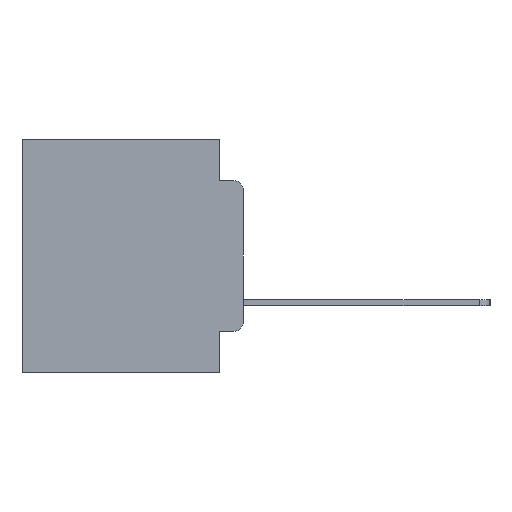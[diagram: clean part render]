
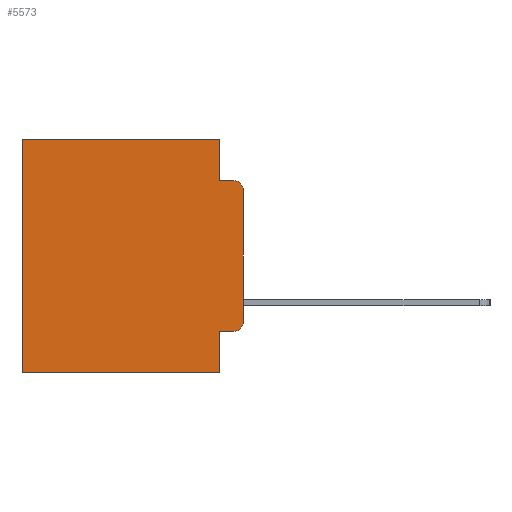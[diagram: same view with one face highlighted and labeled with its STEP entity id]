
A CAD part, left-side view. The second image highlights one B-rep face of the part: STEP entity #5573.
In plain terms, the highlighted planar face has unit normal (-1, 0, 0).
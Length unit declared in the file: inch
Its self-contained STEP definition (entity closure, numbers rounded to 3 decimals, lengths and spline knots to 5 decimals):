
#157 = CARTESIAN_POINT ( 'NONE',  ( 0.298, 0.051, 0. ) ) ;
#373 = DIRECTION ( 'NONE',  ( 0., 0., -1. ) ) ;
#745 = CARTESIAN_POINT ( 'NONE',  ( 0.298, 0., -0.1085 ) ) ;
#975 = EDGE_CURVE ( 'NONE', #8315, #5218, #23896, .T. ) ;
#1308 = CIRCLE ( 'NONE', #10389, 0.02 ) ;
#1466 = EDGE_CURVE ( 'NONE', #11784, #9131, #1308, .T. ) ;
#1642 = ORIENTED_EDGE ( 'NONE', *, *, #18686, .F. ) ;
#1807 = CARTESIAN_POINT ( 'NONE',  ( 0.298, 0., 0. ) ) ;
#1975 = ORIENTED_EDGE ( 'NONE', *, *, #1466, .T. ) ;
#2349 = DIRECTION ( 'NONE',  ( 0., 0., -1. ) ) ;
#2386 = DIRECTION ( 'NONE',  ( 0., 0., -1. ) ) ;
#2549 = DIRECTION ( 'NONE',  ( 0., 1., 0. ) ) ;
#2755 = CARTESIAN_POINT ( 'NONE',  ( 0.298, 0.051, -0.5 ) ) ;
#2875 = VERTEX_POINT ( 'NONE', #2915 ) ;
#2915 = CARTESIAN_POINT ( 'NONE',  ( 0.298, 0.473, 0. ) ) ;
#3082 = VECTOR ( 'NONE', #373, 39.37008 ) ;
#3788 = LINE ( 'NONE', #9701, #3082 ) ;
#4056 = ORIENTED_EDGE ( 'NONE', *, *, #16847, .T. ) ;
#4488 = FACE_OUTER_BOUND ( 'NONE', #4966, .T. ) ;
#4672 = LINE ( 'NONE', #1807, #26357 ) ;
#4964 = VECTOR ( 'NONE', #21212, 39.37008 ) ;
#4966 = EDGE_LOOP ( 'NONE', ( #1642, #4056, #24795, #11337, #16943, #10158, #23869, #9691, #23534, #1975 ) ) ;
#5168 = CARTESIAN_POINT ( 'NONE',  ( 0.298, 0.02, -0.4115 ) ) ;
#5218 = VERTEX_POINT ( 'NONE', #2755 ) ;
#5573 = ADVANCED_FACE ( 'NONE', ( #4488 ), #20817, .F. ) ;
#5608 = EDGE_CURVE ( 'NONE', #2875, #20898, #3788, .T. ) ;
#7096 = VECTOR ( 'NONE', #2386, 39.37008 ) ;
#7436 = VERTEX_POINT ( 'NONE', #745 ) ;
#7667 = LINE ( 'NONE', #21018, #19528 ) ;
#7690 = CARTESIAN_POINT ( 'NONE',  ( 0.298, 0., 0. ) ) ;
#8021 = CARTESIAN_POINT ( 'NONE',  ( 0.298, 0.02, -0.1085 ) ) ;
#8149 = EDGE_CURVE ( 'NONE', #25382, #12255, #17837, .T. ) ;
#8315 = VERTEX_POINT ( 'NONE', #11534 ) ;
#8318 = CARTESIAN_POINT ( 'NONE',  ( 0.298, 0.051, 0. ) ) ;
#9057 = AXIS2_PLACEMENT_3D ( 'NONE', #7690, #13308, #16652 ) ;
#9131 = VERTEX_POINT ( 'NONE', #25264 ) ;
#9298 = VERTEX_POINT ( 'NONE', #13346 ) ;
#9691 = ORIENTED_EDGE ( 'NONE', *, *, #975, .F. ) ;
#9701 = CARTESIAN_POINT ( 'NONE',  ( 0.298, 0.473, 0. ) ) ;
#9945 = LINE ( 'NONE', #27325, #4964 ) ;
#10149 = DIRECTION ( 'NONE',  ( 0., 0., -1. ) ) ;
#10158 = ORIENTED_EDGE ( 'NONE', *, *, #5608, .T. ) ;
#10385 = CARTESIAN_POINT ( 'NONE',  ( 0.298, 0.051, 0. ) ) ;
#10389 = AXIS2_PLACEMENT_3D ( 'NONE', #13475, #18407, #18294 ) ;
#10555 = DIRECTION ( 'NONE',  ( 0., 0., -1. ) ) ;
#11018 = CARTESIAN_POINT ( 'NONE',  ( 0.298, 0.051, -0.0885 ) ) ;
#11337 = ORIENTED_EDGE ( 'NONE', *, *, #8149, .F. ) ;
#11534 = CARTESIAN_POINT ( 'NONE',  ( 0.298, 0.051, -0.4115 ) ) ;
#11784 = VERTEX_POINT ( 'NONE', #5168 ) ;
#12255 = VERTEX_POINT ( 'NONE', #11018 ) ;
#13308 = DIRECTION ( 'NONE',  ( 1., 0., 0. ) ) ;
#13346 = CARTESIAN_POINT ( 'NONE',  ( 0.298, 0.02, -0.0885 ) ) ;
#13475 = CARTESIAN_POINT ( 'NONE',  ( 0.298, 0.02, -0.3915 ) ) ;
#14135 = CIRCLE ( 'NONE', #26826, 0.02 ) ;
#14539 = EDGE_CURVE ( 'NONE', #12255, #9298, #7667, .T. ) ;
#15357 = CARTESIAN_POINT ( 'NONE',  ( 0.298, 0., -0.5 ) ) ;
#16537 = VECTOR ( 'NONE', #2349, 39.37008 ) ;
#16541 = EDGE_CURVE ( 'NONE', #5218, #20898, #17782, .T. ) ;
#16652 = DIRECTION ( 'NONE',  ( 0., 0., -1. ) ) ;
#16847 = EDGE_CURVE ( 'NONE', #7436, #9298, #14135, .T. ) ;
#16943 = ORIENTED_EDGE ( 'NONE', *, *, #26173, .T. ) ;
#17782 = LINE ( 'NONE', #15357, #22057 ) ;
#17837 = LINE ( 'NONE', #157, #16537 ) ;
#18294 = DIRECTION ( 'NONE',  ( 0., 0., -1. ) ) ;
#18407 = DIRECTION ( 'NONE',  ( -1., 0., 0. ) ) ;
#18686 = EDGE_CURVE ( 'NONE', #7436, #9131, #26459, .T. ) ;
#18915 = CARTESIAN_POINT ( 'NONE',  ( 0.298, 0., 0. ) ) ;
#19528 = VECTOR ( 'NONE', #25188, 39.37008 ) ;
#20817 = PLANE ( 'NONE',  #9057 ) ;
#20898 = VERTEX_POINT ( 'NONE', #26015 ) ;
#20923 = DIRECTION ( 'NONE',  ( 0., 1., 0. ) ) ;
#20966 = VECTOR ( 'NONE', #10555, 39.37008 ) ;
#21018 = CARTESIAN_POINT ( 'NONE',  ( 0.298, 0.051, -0.0885 ) ) ;
#21212 = DIRECTION ( 'NONE',  ( 0., -1., 0. ) ) ;
#22057 = VECTOR ( 'NONE', #2549, 39.37008 ) ;
#22754 = DIRECTION ( 'NONE',  ( -1., 0., 0. ) ) ;
#23086 = EDGE_CURVE ( 'NONE', #8315, #11784, #9945, .T. ) ;
#23534 = ORIENTED_EDGE ( 'NONE', *, *, #23086, .T. ) ;
#23869 = ORIENTED_EDGE ( 'NONE', *, *, #16541, .F. ) ;
#23896 = LINE ( 'NONE', #8318, #7096 ) ;
#24795 = ORIENTED_EDGE ( 'NONE', *, *, #14539, .F. ) ;
#25188 = DIRECTION ( 'NONE',  ( 0., -1., 0. ) ) ;
#25264 = CARTESIAN_POINT ( 'NONE',  ( 0.298, 0., -0.3915 ) ) ;
#25382 = VERTEX_POINT ( 'NONE', #10385 ) ;
#26015 = CARTESIAN_POINT ( 'NONE',  ( 0.298, 0.473, -0.5 ) ) ;
#26173 = EDGE_CURVE ( 'NONE', #25382, #2875, #4672, .T. ) ;
#26357 = VECTOR ( 'NONE', #20923, 39.37008 ) ;
#26459 = LINE ( 'NONE', #18915, #20966 ) ;
#26826 = AXIS2_PLACEMENT_3D ( 'NONE', #8021, #22754, #10149 ) ;
#27325 = CARTESIAN_POINT ( 'NONE',  ( 0.298, 0.051, -0.4115 ) ) ;
